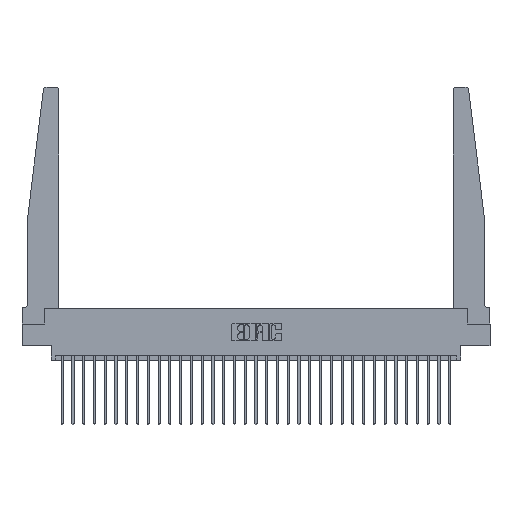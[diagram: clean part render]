
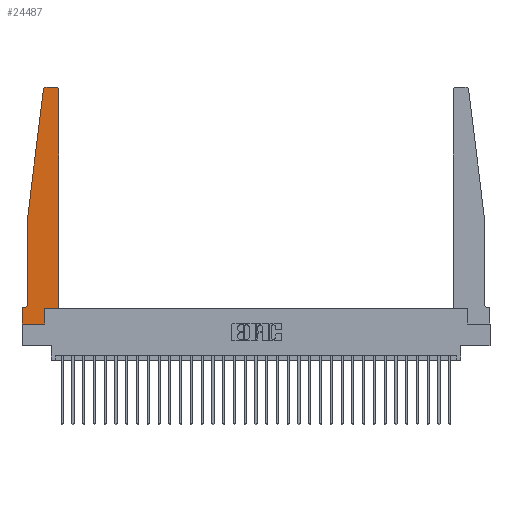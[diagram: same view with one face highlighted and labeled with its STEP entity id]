
A CAD part, top view. The second image highlights one B-rep face of the part: STEP entity #24487.
In plain terms, the highlighted planar face has unit normal (0, 0, 1).
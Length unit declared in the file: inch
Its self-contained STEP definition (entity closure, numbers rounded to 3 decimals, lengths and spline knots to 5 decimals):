
#362 = VERTEX_POINT ( 'NONE', #16535 ) ;
#407 = CARTESIAN_POINT ( 'NONE',  ( 0.065, 1.25, 0.37 ) ) ;
#603 = DIRECTION ( 'NONE',  ( 0., 0., 1. ) ) ;
#1014 = CARTESIAN_POINT ( 'NONE',  ( 0., 0., 0.37 ) ) ;
#1301 = VECTOR ( 'NONE', #4459, 39.37008 ) ;
#1433 = LINE ( 'NONE', #11092, #19818 ) ;
#1738 = DIRECTION ( 'NONE',  ( -0.122, -0.992, 0. ) ) ;
#1779 = ORIENTED_EDGE ( 'NONE', *, *, #22105, .T. ) ;
#1933 = VERTEX_POINT ( 'NONE', #22471 ) ;
#2586 = LINE ( 'NONE', #15031, #20226 ) ;
#2793 = AXIS2_PLACEMENT_3D ( 'NONE', #3025, #19120, #5338 ) ;
#2913 = DIRECTION ( 'NONE',  ( -1., 0., 0. ) ) ;
#3025 = CARTESIAN_POINT ( 'NONE',  ( 0.395, 2.72, 0.37 ) ) ;
#3182 = CARTESIAN_POINT ( 'NONE',  ( 0.425, 2.72, 0.37 ) ) ;
#3526 = VERTEX_POINT ( 'NONE', #3182 ) ;
#3982 = ORIENTED_EDGE ( 'NONE', *, *, #5979, .T. ) ;
#4459 = DIRECTION ( 'NONE',  ( 1., 0., 0. ) ) ;
#4736 = VECTOR ( 'NONE', #12286, 39.37008 ) ;
#4744 = CARTESIAN_POINT ( 'NONE',  ( 0., 0., 0.37 ) ) ;
#5338 = DIRECTION ( 'NONE',  ( 1., 0., 0. ) ) ;
#5374 = CARTESIAN_POINT ( 'NONE',  ( 0.015, 0.2375, 0.37 ) ) ;
#5422 = VERTEX_POINT ( 'NONE', #17290 ) ;
#5632 = EDGE_CURVE ( 'NONE', #5422, #20170, #1433, .T. ) ;
#5979 = EDGE_CURVE ( 'NONE', #10757, #5422, #11241, .T. ) ;
#6730 = LINE ( 'NONE', #18259, #1301 ) ;
#6749 = PLANE ( 'NONE',  #19695 ) ;
#6943 = VERTEX_POINT ( 'NONE', #14614 ) ;
#7058 = CARTESIAN_POINT ( 'NONE',  ( 0.27653, 2.75, 0.37 ) ) ;
#7446 = DIRECTION ( 'NONE',  ( 0., 1., 0. ) ) ;
#7695 = DIRECTION ( 'NONE',  ( -1., 0., 0. ) ) ;
#8659 = LINE ( 'NONE', #23528, #26198 ) ;
#9029 = CARTESIAN_POINT ( 'NONE',  ( 0., 0., 0.37 ) ) ;
#9117 = DIRECTION ( 'NONE',  ( 0., 0., 1. ) ) ;
#9814 = LINE ( 'NONE', #29552, #14489 ) ;
#9962 = CARTESIAN_POINT ( 'NONE',  ( 0.2605, 0.18, 0.37 ) ) ;
#10095 = AXIS2_PLACEMENT_3D ( 'NONE', #5374, #21468, #7695 ) ;
#10757 = VERTEX_POINT ( 'NONE', #7058 ) ;
#10907 = EDGE_CURVE ( 'NONE', #3526, #29039, #23850, .T. ) ;
#10911 = VECTOR ( 'NONE', #11374, 39.37008 ) ;
#10945 = ORIENTED_EDGE ( 'NONE', *, *, #25801, .T. ) ;
#11092 = CARTESIAN_POINT ( 'NONE',  ( 0.065, 1.25, 0.37 ) ) ;
#11241 = CIRCLE ( 'NONE', #24849, 0.03 ) ;
#11372 = CARTESIAN_POINT ( 'NONE',  ( 0., 0.1875, 0.37 ) ) ;
#11374 = DIRECTION ( 'NONE',  ( 1., 0., 0. ) ) ;
#11606 = ORIENTED_EDGE ( 'NONE', *, *, #17024, .T. ) ;
#12286 = DIRECTION ( 'NONE',  ( 0., 1., 0. ) ) ;
#13671 = CARTESIAN_POINT ( 'NONE',  ( 0.395, 2.75, 0.37 ) ) ;
#14341 = CARTESIAN_POINT ( 'NONE',  ( 0.065, 0.1875, 0.37 ) ) ;
#14469 = CARTESIAN_POINT ( 'NONE',  ( 0.27653, 2.72, 0.37 ) ) ;
#14489 = VECTOR ( 'NONE', #22715, 39.37008 ) ;
#14614 = CARTESIAN_POINT ( 'NONE',  ( 0.2605, 0.18, 0.37 ) ) ;
#14999 = CARTESIAN_POINT ( 'NONE',  ( 0.015, 0.1875, 0.37 ) ) ;
#15031 = CARTESIAN_POINT ( 'NONE',  ( 0.25, 2.75, 0.37 ) ) ;
#15184 = EDGE_CURVE ( 'NONE', #20170, #1933, #9814, .T. ) ;
#15321 = EDGE_CURVE ( 'NONE', #28090, #362, #29109, .T. ) ;
#15421 = VERTEX_POINT ( 'NONE', #11372 ) ;
#15929 = ORIENTED_EDGE ( 'NONE', *, *, #24726, .T. ) ;
#16242 = ORIENTED_EDGE ( 'NONE', *, *, #5632, .T. ) ;
#16535 = CARTESIAN_POINT ( 'NONE',  ( 0.2605, 0., 0.37 ) ) ;
#16769 = DIRECTION ( 'NONE',  ( 1., 0., 0. ) ) ;
#17017 = LINE ( 'NONE', #9962, #4736 ) ;
#17024 = EDGE_CURVE ( 'NONE', #1933, #27565, #22624, .T. ) ;
#17290 = CARTESIAN_POINT ( 'NONE',  ( 0.24675, 2.72367, 0.37 ) ) ;
#17333 = DIRECTION ( 'NONE',  ( -1., 0., 0. ) ) ;
#17411 = VECTOR ( 'NONE', #18525, 39.37008 ) ;
#18259 = CARTESIAN_POINT ( 'NONE',  ( 0.425, 0.18, 0.37 ) ) ;
#18525 = DIRECTION ( 'NONE',  ( 0., -1., 0. ) ) ;
#18735 = ORIENTED_EDGE ( 'NONE', *, *, #21793, .T. ) ;
#18925 = EDGE_CURVE ( 'NONE', #27565, #15421, #26851, .T. ) ;
#19120 = DIRECTION ( 'NONE',  ( 0., 0., 1. ) ) ;
#19695 = AXIS2_PLACEMENT_3D ( 'NONE', #22852, #9117, #25130 ) ;
#19781 = FACE_OUTER_BOUND ( 'NONE', #24055, .T. ) ;
#19818 = VECTOR ( 'NONE', #1738, 39.37008 ) ;
#20170 = VERTEX_POINT ( 'NONE', #407 ) ;
#20226 = VECTOR ( 'NONE', #17333, 39.37008 ) ;
#21468 = DIRECTION ( 'NONE',  ( 0., 0., -1. ) ) ;
#21636 = ORIENTED_EDGE ( 'NONE', *, *, #15321, .T. ) ;
#21793 = EDGE_CURVE ( 'NONE', #15421, #28090, #29529, .T. ) ;
#22105 = EDGE_CURVE ( 'NONE', #29039, #10757, #2586, .T. ) ;
#22471 = CARTESIAN_POINT ( 'NONE',  ( 0.065, 0.2375, 0.37 ) ) ;
#22624 = CIRCLE ( 'NONE', #10095, 0.05 ) ;
#22715 = DIRECTION ( 'NONE',  ( 0., -1., 0. ) ) ;
#22852 = CARTESIAN_POINT ( 'NONE',  ( 0., 0.1875, 0.37 ) ) ;
#23202 = EDGE_CURVE ( 'NONE', #362, #6943, #17017, .T. ) ;
#23412 = ORIENTED_EDGE ( 'NONE', *, *, #18925, .T. ) ;
#23528 = CARTESIAN_POINT ( 'NONE',  ( 0.425, 0.18, 0.37 ) ) ;
#23850 = CIRCLE ( 'NONE', #2793, 0.03 ) ;
#23938 = CARTESIAN_POINT ( 'NONE',  ( 0.425, 0.18, 0.37 ) ) ;
#24055 = EDGE_LOOP ( 'NONE', ( #1779, #3982, #16242, #28740, #11606, #23412, #18735, #21636, #26641, #10945, #15929, #25568 ) ) ;
#24487 = ADVANCED_FACE ( 'NONE', ( #19781 ), #6749, .T. ) ;
#24726 = EDGE_CURVE ( 'NONE', #26153, #3526, #8659, .T. ) ;
#24849 = AXIS2_PLACEMENT_3D ( 'NONE', #14469, #603, #16769 ) ;
#25130 = DIRECTION ( 'NONE',  ( 1., 0., 0. ) ) ;
#25568 = ORIENTED_EDGE ( 'NONE', *, *, #10907, .T. ) ;
#25801 = EDGE_CURVE ( 'NONE', #6943, #26153, #6730, .T. ) ;
#26125 = VECTOR ( 'NONE', #2913, 39.37008 ) ;
#26153 = VERTEX_POINT ( 'NONE', #23938 ) ;
#26198 = VECTOR ( 'NONE', #7446, 39.37008 ) ;
#26641 = ORIENTED_EDGE ( 'NONE', *, *, #23202, .T. ) ;
#26851 = LINE ( 'NONE', #14341, #26125 ) ;
#27565 = VERTEX_POINT ( 'NONE', #14999 ) ;
#28090 = VERTEX_POINT ( 'NONE', #1014 ) ;
#28740 = ORIENTED_EDGE ( 'NONE', *, *, #15184, .T. ) ;
#29039 = VERTEX_POINT ( 'NONE', #13671 ) ;
#29109 = LINE ( 'NONE', #9029, #10911 ) ;
#29529 = LINE ( 'NONE', #4744, #17411 ) ;
#29552 = CARTESIAN_POINT ( 'NONE',  ( 0.065, 1.25, 0.37 ) ) ;
